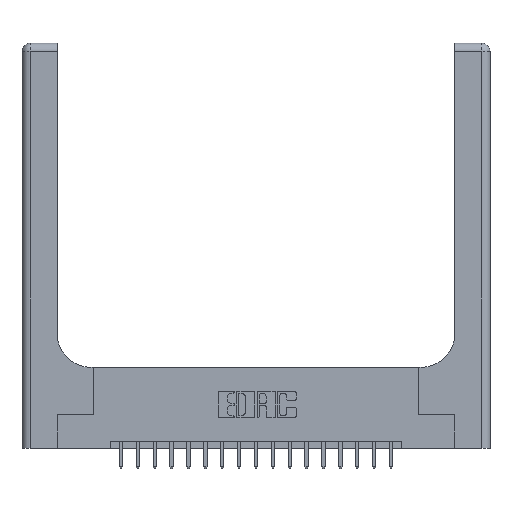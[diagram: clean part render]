
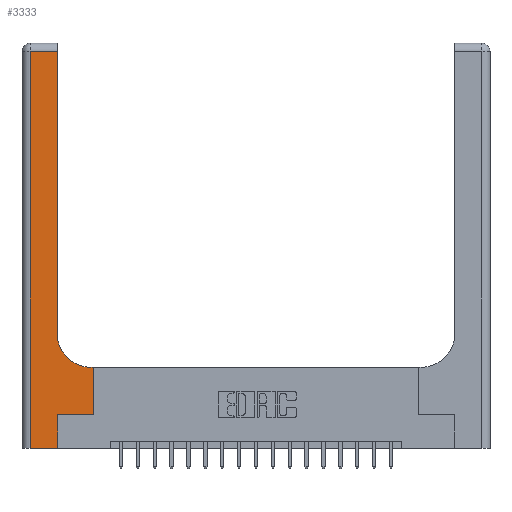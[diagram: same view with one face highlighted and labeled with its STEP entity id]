
A CAD part, top view. The second image highlights one B-rep face of the part: STEP entity #3333.
In plain terms, the highlighted planar face has unit normal (0, 0, 1).
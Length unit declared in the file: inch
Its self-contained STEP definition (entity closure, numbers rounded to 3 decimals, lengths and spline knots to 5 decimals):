
#68 = CARTESIAN_POINT ( 'NONE',  ( 0.51, 0.85, 0.37 ) ) ;
#207 = LINE ( 'NONE', #4440, #5701 ) ;
#241 = CARTESIAN_POINT ( 'NONE',  ( 0.06, 3., 0.37 ) ) ;
#411 = VERTEX_POINT ( 'NONE', #1399 ) ;
#535 = EDGE_CURVE ( 'NONE', #5036, #807, #13982, .T. ) ;
#684 = CARTESIAN_POINT ( 'NONE',  ( 0., 3., 0.37 ) ) ;
#807 = VERTEX_POINT ( 'NONE', #17094 ) ;
#1274 = CARTESIAN_POINT ( 'NONE',  ( 0.528, 0.25, 0.37 ) ) ;
#1399 = CARTESIAN_POINT ( 'NONE',  ( 0.26, 2.94, 0.37 ) ) ;
#1597 = DIRECTION ( 'NONE',  ( 0., 0., -1. ) ) ;
#2396 = EDGE_CURVE ( 'NONE', #8724, #411, #4732, .T. ) ;
#2474 = EDGE_CURVE ( 'NONE', #16049, #8724, #16797, .T. ) ;
#2522 = VECTOR ( 'NONE', #9649, 39.37008 ) ;
#2818 = EDGE_CURVE ( 'NONE', #10282, #16049, #7588, .T. ) ;
#3333 = ADVANCED_FACE ( 'NONE', ( #8269 ), #12937, .F. ) ;
#3883 = VECTOR ( 'NONE', #10454, 39.37008 ) ;
#3994 = DIRECTION ( 'NONE',  ( 1., 0., 0. ) ) ;
#4249 = AXIS2_PLACEMENT_3D ( 'NONE', #68, #1597, #9172 ) ;
#4440 = CARTESIAN_POINT ( 'NONE',  ( 0.528, 0.25, 0.37 ) ) ;
#4732 = LINE ( 'NONE', #8645, #7605 ) ;
#5036 = VERTEX_POINT ( 'NONE', #8273 ) ;
#5056 = ORIENTED_EDGE ( 'NONE', *, *, #2474, .T. ) ;
#5236 = ORIENTED_EDGE ( 'NONE', *, *, #17896, .T. ) ;
#5360 = ORIENTED_EDGE ( 'NONE', *, *, #6019, .T. ) ;
#5701 = VECTOR ( 'NONE', #10383, 39.37008 ) ;
#5878 = ORIENTED_EDGE ( 'NONE', *, *, #2396, .T. ) ;
#5988 = CARTESIAN_POINT ( 'NONE',  ( 0., 2.94, 0.37 ) ) ;
#6019 = EDGE_CURVE ( 'NONE', #411, #5036, #15688, .T. ) ;
#7293 = EDGE_CURVE ( 'NONE', #16226, #12249, #15752, .T. ) ;
#7540 = EDGE_LOOP ( 'NONE', ( #5878, #5360, #17914, #5236, #19632, #8300, #19295, #16214, #5056 ) ) ;
#7564 = CARTESIAN_POINT ( 'NONE',  ( 0.51, 0.6, 0.37 ) ) ;
#7588 = LINE ( 'NONE', #18349, #17249 ) ;
#7605 = VECTOR ( 'NONE', #11740, 39.37008 ) ;
#8269 = FACE_OUTER_BOUND ( 'NONE', #7540, .T. ) ;
#8273 = CARTESIAN_POINT ( 'NONE',  ( 0.06, 2.94, 0.37 ) ) ;
#8300 = ORIENTED_EDGE ( 'NONE', *, *, #9026, .T. ) ;
#8314 = VERTEX_POINT ( 'NONE', #1274 ) ;
#8393 = DIRECTION ( 'NONE',  ( -1., 0., 0. ) ) ;
#8645 = CARTESIAN_POINT ( 'NONE',  ( 0.26, 3., 0.37 ) ) ;
#8677 = CARTESIAN_POINT ( 'NONE',  ( 0.528, 0.6, 0.37 ) ) ;
#8724 = VERTEX_POINT ( 'NONE', #15579 ) ;
#9026 = EDGE_CURVE ( 'NONE', #12249, #8314, #15681, .T. ) ;
#9172 = DIRECTION ( 'NONE',  ( 1., 0., 0. ) ) ;
#9536 = DIRECTION ( 'NONE',  ( 0., -1., 0. ) ) ;
#9649 = DIRECTION ( 'NONE',  ( 0., 1., 0. ) ) ;
#10282 = VERTEX_POINT ( 'NONE', #8677 ) ;
#10383 = DIRECTION ( 'NONE',  ( 0., 1., 0. ) ) ;
#10454 = DIRECTION ( 'NONE',  ( -1., 0., 0. ) ) ;
#10805 = EDGE_CURVE ( 'NONE', #8314, #10282, #207, .T. ) ;
#11740 = DIRECTION ( 'NONE',  ( 0., 1., 0. ) ) ;
#11746 = CARTESIAN_POINT ( 'NONE',  ( 0., 0., 0.37 ) ) ;
#12109 = VECTOR ( 'NONE', #9536, 39.37008 ) ;
#12177 = DIRECTION ( 'NONE',  ( -1., 0., 0. ) ) ;
#12249 = VERTEX_POINT ( 'NONE', #12271 ) ;
#12271 = CARTESIAN_POINT ( 'NONE',  ( 0.265, 0.25, 0.37 ) ) ;
#12937 = PLANE ( 'NONE',  #16946 ) ;
#13982 = LINE ( 'NONE', #241, #12109 ) ;
#14472 = CARTESIAN_POINT ( 'NONE',  ( 0.265, 0.25, 0.37 ) ) ;
#15035 = DIRECTION ( 'NONE',  ( 1., 0., 0. ) ) ;
#15579 = CARTESIAN_POINT ( 'NONE',  ( 0.26, 0.85, 0.37 ) ) ;
#15681 = LINE ( 'NONE', #14472, #18102 ) ;
#15688 = LINE ( 'NONE', #5988, #3883 ) ;
#15752 = LINE ( 'NONE', #18740, #2522 ) ;
#16049 = VERTEX_POINT ( 'NONE', #7564 ) ;
#16214 = ORIENTED_EDGE ( 'NONE', *, *, #2818, .T. ) ;
#16226 = VERTEX_POINT ( 'NONE', #18524 ) ;
#16797 = CIRCLE ( 'NONE', #4249, 0.25 ) ;
#16946 = AXIS2_PLACEMENT_3D ( 'NONE', #684, #17391, #8393 ) ;
#17094 = CARTESIAN_POINT ( 'NONE',  ( 0.06, 0., 0.37 ) ) ;
#17249 = VECTOR ( 'NONE', #12177, 39.37008 ) ;
#17391 = DIRECTION ( 'NONE',  ( 0., 0., -1. ) ) ;
#17896 = EDGE_CURVE ( 'NONE', #807, #16226, #18435, .T. ) ;
#17914 = ORIENTED_EDGE ( 'NONE', *, *, #535, .T. ) ;
#17969 = VECTOR ( 'NONE', #15035, 39.37008 ) ;
#18102 = VECTOR ( 'NONE', #3994, 39.37008 ) ;
#18349 = CARTESIAN_POINT ( 'NONE',  ( 0.26, 0.6, 0.37 ) ) ;
#18435 = LINE ( 'NONE', #11746, #17969 ) ;
#18524 = CARTESIAN_POINT ( 'NONE',  ( 0.265, 0., 0.37 ) ) ;
#18740 = CARTESIAN_POINT ( 'NONE',  ( 0.265, 0., 0.37 ) ) ;
#19295 = ORIENTED_EDGE ( 'NONE', *, *, #10805, .T. ) ;
#19632 = ORIENTED_EDGE ( 'NONE', *, *, #7293, .T. ) ;
